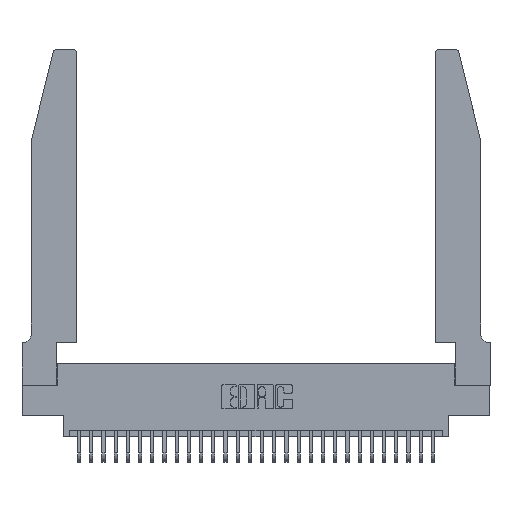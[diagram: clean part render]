
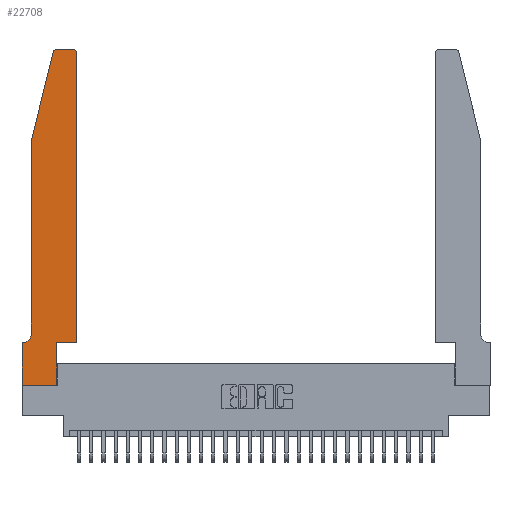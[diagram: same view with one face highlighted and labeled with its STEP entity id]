
A CAD part, top view. The second image highlights one B-rep face of the part: STEP entity #22708.
In plain terms, the highlighted planar face has unit normal (0, 0, 1).
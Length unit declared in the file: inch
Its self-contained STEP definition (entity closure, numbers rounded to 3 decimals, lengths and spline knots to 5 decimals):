
#124 = CARTESIAN_POINT ( 'NONE',  ( 0.0755, 0.35, 0.37 ) ) ;
#515 = LINE ( 'NONE', #124, #3988 ) ;
#704 = LINE ( 'NONE', #13890, #26413 ) ;
#945 = VERTEX_POINT ( 'NONE', #23300 ) ;
#1261 = VECTOR ( 'NONE', #24313, 39.37008 ) ;
#1283 = EDGE_CURVE ( 'NONE', #945, #6335, #515, .T. ) ;
#1445 = EDGE_CURVE ( 'NONE', #8140, #25328, #18498, .T. ) ;
#1469 = VERTEX_POINT ( 'NONE', #25350 ) ;
#1696 = LINE ( 'NONE', #6607, #10823 ) ;
#2645 = CARTESIAN_POINT ( 'NONE',  ( 0.4505, 0.35, 0.37 ) ) ;
#3176 = VECTOR ( 'NONE', #12551, 39.37008 ) ;
#3988 = VECTOR ( 'NONE', #8344, 39.37008 ) ;
#4131 = AXIS2_PLACEMENT_3D ( 'NONE', #28337, #13633, #30762 ) ;
#4181 = DIRECTION ( 'NONE',  ( 0., 1., 0. ) ) ;
#4407 = DIRECTION ( 'NONE',  ( 0., 0., 1. ) ) ;
#4426 = EDGE_CURVE ( 'NONE', #6283, #8140, #31699, .T. ) ;
#4821 = CARTESIAN_POINT ( 'NONE',  ( 0.4205, 2.72, 0.37 ) ) ;
#4868 = VERTEX_POINT ( 'NONE', #8003 ) ;
#5028 = VERTEX_POINT ( 'NONE', #8995 ) ;
#5665 = CARTESIAN_POINT ( 'NONE',  ( 0.284, 2.72, 0.37 ) ) ;
#6283 = VERTEX_POINT ( 'NONE', #25091 ) ;
#6335 = VERTEX_POINT ( 'NONE', #22804 ) ;
#6607 = CARTESIAN_POINT ( 'NONE',  ( 0.2605, 2.75, 0.37 ) ) ;
#6815 = AXIS2_PLACEMENT_3D ( 'NONE', #5665, #8144, #25633 ) ;
#7067 = CARTESIAN_POINT ( 'NONE',  ( 0., 0., 0.37 ) ) ;
#7292 = EDGE_CURVE ( 'NONE', #5028, #26069, #12222, .T. ) ;
#7722 = ORIENTED_EDGE ( 'NONE', *, *, #1283, .T. ) ;
#8003 = CARTESIAN_POINT ( 'NONE',  ( 0.284, 2.75, 0.37 ) ) ;
#8140 = VERTEX_POINT ( 'NONE', #10508 ) ;
#8144 = DIRECTION ( 'NONE',  ( 0., 0., 1. ) ) ;
#8344 = DIRECTION ( 'NONE',  ( -1., 0., 0. ) ) ;
#8589 = FACE_OUTER_BOUND ( 'NONE', #10371, .T. ) ;
#8700 = CIRCLE ( 'NONE', #4131, 0.07 ) ;
#8768 = CARTESIAN_POINT ( 'NONE',  ( 0.0755, 0.42, 0.37 ) ) ;
#8975 = EDGE_CURVE ( 'NONE', #9098, #945, #8700, .T. ) ;
#8995 = CARTESIAN_POINT ( 'NONE',  ( 0.25487, 2.72718, 0.37 ) ) ;
#9098 = VERTEX_POINT ( 'NONE', #8768 ) ;
#9481 = DIRECTION ( 'NONE',  ( 1., 0., 0. ) ) ;
#9803 = DIRECTION ( 'NONE',  ( -0.239, -0.971, 0. ) ) ;
#10371 = EDGE_LOOP ( 'NONE', ( #22813, #12499, #15343, #17053, #26474, #7722, #26933, #31411, #22785, #14251, #28857, #16248 ) ) ;
#10508 = CARTESIAN_POINT ( 'NONE',  ( 0.4505, 0.35, 0.37 ) ) ;
#10823 = VECTOR ( 'NONE', #28600, 39.37008 ) ;
#11588 = LINE ( 'NONE', #7067, #1261 ) ;
#11736 = EDGE_CURVE ( 'NONE', #15132, #4868, #1696, .T. ) ;
#11779 = AXIS2_PLACEMENT_3D ( 'NONE', #4821, #4407, #26479 ) ;
#12222 = LINE ( 'NONE', #19566, #19533 ) ;
#12229 = CARTESIAN_POINT ( 'NONE',  ( 0., 0., 0.37 ) ) ;
#12390 = VERTEX_POINT ( 'NONE', #17579 ) ;
#12469 = EDGE_CURVE ( 'NONE', #4868, #5028, #27349, .T. ) ;
#12499 = ORIENTED_EDGE ( 'NONE', *, *, #12469, .T. ) ;
#12551 = DIRECTION ( 'NONE',  ( 0., -1., 0. ) ) ;
#12725 = VECTOR ( 'NONE', #22212, 39.37008 ) ;
#13633 = DIRECTION ( 'NONE',  ( 0., 0., -1. ) ) ;
#13890 = CARTESIAN_POINT ( 'NONE',  ( 0.2865, 0.35, 0.37 ) ) ;
#13952 = CARTESIAN_POINT ( 'NONE',  ( 0.4505, 2.72, 0.37 ) ) ;
#14251 = ORIENTED_EDGE ( 'NONE', *, *, #4426, .T. ) ;
#15132 = VERTEX_POINT ( 'NONE', #18195 ) ;
#15305 = EDGE_CURVE ( 'NONE', #25328, #15132, #28284, .T. ) ;
#15343 = ORIENTED_EDGE ( 'NONE', *, *, #7292, .T. ) ;
#16173 = LINE ( 'NONE', #12229, #3176 ) ;
#16248 = ORIENTED_EDGE ( 'NONE', *, *, #15305, .T. ) ;
#17053 = ORIENTED_EDGE ( 'NONE', *, *, #21863, .T. ) ;
#17089 = CARTESIAN_POINT ( 'NONE',  ( 0., 0.35, 0.37 ) ) ;
#17579 = CARTESIAN_POINT ( 'NONE',  ( 0.2865, 0., 0.37 ) ) ;
#18195 = CARTESIAN_POINT ( 'NONE',  ( 0.4205, 2.75, 0.37 ) ) ;
#18498 = LINE ( 'NONE', #2645, #12725 ) ;
#19239 = PLANE ( 'NONE',  #30774 ) ;
#19366 = DIRECTION ( 'NONE',  ( 0., -1., 0. ) ) ;
#19533 = VECTOR ( 'NONE', #9803, 39.37008 ) ;
#19566 = CARTESIAN_POINT ( 'NONE',  ( 0.0755, 2., 0.37 ) ) ;
#20102 = LINE ( 'NONE', #26482, #24736 ) ;
#20483 = EDGE_CURVE ( 'NONE', #12390, #6283, #704, .T. ) ;
#21863 = EDGE_CURVE ( 'NONE', #26069, #9098, #20102, .T. ) ;
#21886 = CARTESIAN_POINT ( 'NONE',  ( 0.4505, 0.35, 0.37 ) ) ;
#22212 = DIRECTION ( 'NONE',  ( 0., 1., 0. ) ) ;
#22708 = ADVANCED_FACE ( 'NONE', ( #8589 ), #19239, .T. ) ;
#22785 = ORIENTED_EDGE ( 'NONE', *, *, #20483, .T. ) ;
#22804 = CARTESIAN_POINT ( 'NONE',  ( 0., 0.35, 0.37 ) ) ;
#22813 = ORIENTED_EDGE ( 'NONE', *, *, #11736, .T. ) ;
#23300 = CARTESIAN_POINT ( 'NONE',  ( 0.0055, 0.35, 0.37 ) ) ;
#23893 = EDGE_CURVE ( 'NONE', #1469, #12390, #11588, .T. ) ;
#24313 = DIRECTION ( 'NONE',  ( 1., 0., 0. ) ) ;
#24440 = VECTOR ( 'NONE', #31430, 39.37008 ) ;
#24478 = DIRECTION ( 'NONE',  ( 0., 0., 1. ) ) ;
#24736 = VECTOR ( 'NONE', #19366, 39.37008 ) ;
#25091 = CARTESIAN_POINT ( 'NONE',  ( 0.2865, 0.35, 0.37 ) ) ;
#25328 = VERTEX_POINT ( 'NONE', #13952 ) ;
#25350 = CARTESIAN_POINT ( 'NONE',  ( 0., 0., 0.37 ) ) ;
#25633 = DIRECTION ( 'NONE',  ( 1., 0., 0. ) ) ;
#26069 = VERTEX_POINT ( 'NONE', #31356 ) ;
#26413 = VECTOR ( 'NONE', #4181, 39.37008 ) ;
#26474 = ORIENTED_EDGE ( 'NONE', *, *, #8975, .T. ) ;
#26479 = DIRECTION ( 'NONE',  ( 1., 0., 0. ) ) ;
#26482 = CARTESIAN_POINT ( 'NONE',  ( 0.0755, 2., 0.37 ) ) ;
#26933 = ORIENTED_EDGE ( 'NONE', *, *, #27951, .T. ) ;
#27349 = CIRCLE ( 'NONE', #6815, 0.03 ) ;
#27951 = EDGE_CURVE ( 'NONE', #6335, #1469, #16173, .T. ) ;
#28284 = CIRCLE ( 'NONE', #11779, 0.03 ) ;
#28337 = CARTESIAN_POINT ( 'NONE',  ( 0.0055, 0.42, 0.37 ) ) ;
#28600 = DIRECTION ( 'NONE',  ( -1., 0., 0. ) ) ;
#28857 = ORIENTED_EDGE ( 'NONE', *, *, #1445, .T. ) ;
#30762 = DIRECTION ( 'NONE',  ( -1., 0., 0. ) ) ;
#30774 = AXIS2_PLACEMENT_3D ( 'NONE', #17089, #24478, #9481 ) ;
#31356 = CARTESIAN_POINT ( 'NONE',  ( 0.0755, 2., 0.37 ) ) ;
#31411 = ORIENTED_EDGE ( 'NONE', *, *, #23893, .T. ) ;
#31430 = DIRECTION ( 'NONE',  ( 1., 0., 0. ) ) ;
#31699 = LINE ( 'NONE', #21886, #24440 ) ;
